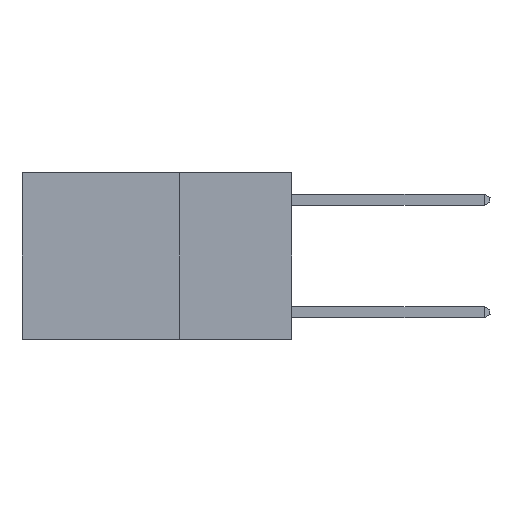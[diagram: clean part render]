
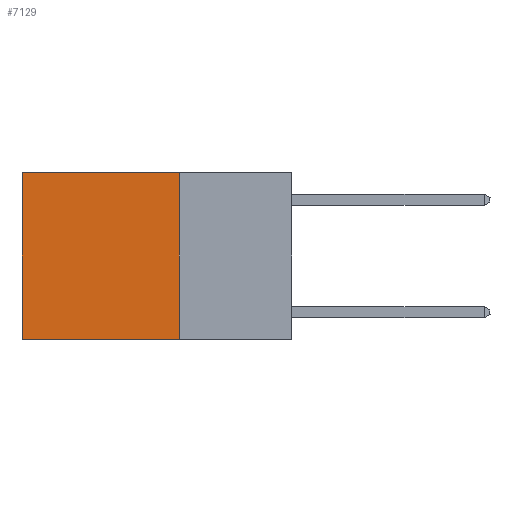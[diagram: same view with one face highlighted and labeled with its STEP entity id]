
A CAD part, left-side view. The second image highlights one B-rep face of the part: STEP entity #7129.
In plain terms, the highlighted planar face has unit normal (-1, 0, 0).
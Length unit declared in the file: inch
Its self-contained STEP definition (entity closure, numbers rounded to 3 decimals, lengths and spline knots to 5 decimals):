
#431 = VERTEX_POINT ( 'NONE', #20327 ) ;
#1928 = FACE_OUTER_BOUND ( 'NONE', #12555, .T. ) ;
#3117 = DIRECTION ( 'NONE',  ( 0., 1., 0. ) ) ;
#3246 = LINE ( 'NONE', #13005, #6055 ) ;
#3547 = DIRECTION ( 'NONE',  ( 0., 1., 0. ) ) ;
#3834 = CARTESIAN_POINT ( 'NONE',  ( 0.2625, 0.25, 0. ) ) ;
#4073 = CARTESIAN_POINT ( 'NONE',  ( 0.2625, 0.25, -0.37 ) ) ;
#4797 = CARTESIAN_POINT ( 'NONE',  ( 0.2625, 0.25, -0.37 ) ) ;
#5537 = VERTEX_POINT ( 'NONE', #4073 ) ;
#6055 = VECTOR ( 'NONE', #11550, 39.37008 ) ;
#6496 = CARTESIAN_POINT ( 'NONE',  ( 0.2625, 0.6, -0.37 ) ) ;
#6872 = PLANE ( 'NONE',  #14765 ) ;
#7129 = ADVANCED_FACE ( 'NONE', ( #1928 ), #6872, .F. ) ;
#7593 = CARTESIAN_POINT ( 'NONE',  ( 0.2625, 0.25, 0. ) ) ;
#7905 = ORIENTED_EDGE ( 'NONE', *, *, #16588, .T. ) ;
#8163 = EDGE_CURVE ( 'NONE', #5537, #15107, #20171, .T. ) ;
#8215 = ORIENTED_EDGE ( 'NONE', *, *, #8860, .T. ) ;
#8701 = ORIENTED_EDGE ( 'NONE', *, *, #8163, .F. ) ;
#8860 = EDGE_CURVE ( 'NONE', #14775, #431, #18919, .T. ) ;
#11467 = VECTOR ( 'NONE', #16435, 39.37008 ) ;
#11550 = DIRECTION ( 'NONE',  ( 0., 0., -1. ) ) ;
#11808 = DIRECTION ( 'NONE',  ( 0., 0., -1. ) ) ;
#12555 = EDGE_LOOP ( 'NONE', ( #7905, #8701, #21770, #8215 ) ) ;
#13005 = CARTESIAN_POINT ( 'NONE',  ( 0.2625, 0.6, 0. ) ) ;
#14765 = AXIS2_PLACEMENT_3D ( 'NONE', #15735, #20439, #11808 ) ;
#14775 = VERTEX_POINT ( 'NONE', #3834 ) ;
#14808 = VECTOR ( 'NONE', #3547, 39.37008 ) ;
#14881 = LINE ( 'NONE', #7593, #11467 ) ;
#15107 = VERTEX_POINT ( 'NONE', #6496 ) ;
#15735 = CARTESIAN_POINT ( 'NONE',  ( 0.2625, 0.25, 0. ) ) ;
#16435 = DIRECTION ( 'NONE',  ( 0., 0., -1. ) ) ;
#16588 = EDGE_CURVE ( 'NONE', #431, #15107, #3246, .T. ) ;
#18193 = EDGE_CURVE ( 'NONE', #14775, #5537, #14881, .T. ) ;
#18919 = LINE ( 'NONE', #19136, #14808 ) ;
#19136 = CARTESIAN_POINT ( 'NONE',  ( 0.2625, 0.25, 0. ) ) ;
#20171 = LINE ( 'NONE', #4797, #20874 ) ;
#20327 = CARTESIAN_POINT ( 'NONE',  ( 0.2625, 0.6, 0. ) ) ;
#20439 = DIRECTION ( 'NONE',  ( 1., 0., 0. ) ) ;
#20874 = VECTOR ( 'NONE', #3117, 39.37008 ) ;
#21770 = ORIENTED_EDGE ( 'NONE', *, *, #18193, .F. ) ;
